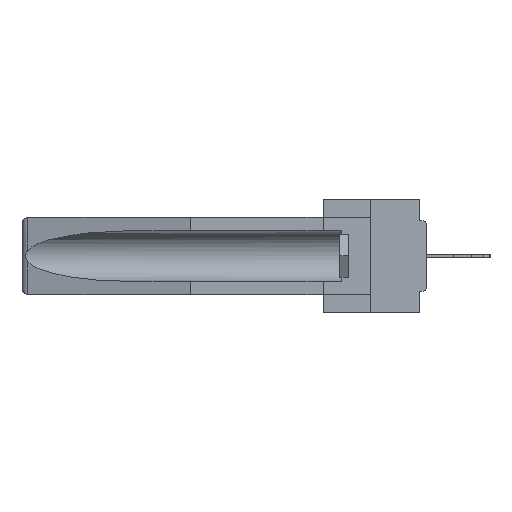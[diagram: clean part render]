
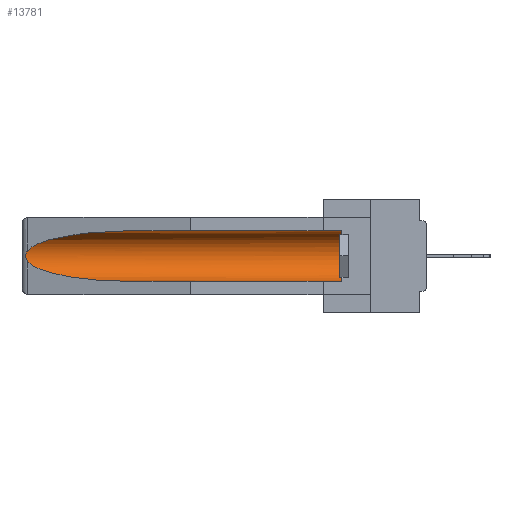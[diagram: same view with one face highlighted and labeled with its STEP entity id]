
A CAD part, left-side view. The second image highlights one B-rep face of the part: STEP entity #13781.
In plain terms, the highlighted cylindrical face has radius 2.857 mm (diameter 5.715 mm), a partial arc.
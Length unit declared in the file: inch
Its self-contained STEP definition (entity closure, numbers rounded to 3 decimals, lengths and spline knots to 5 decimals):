
#148 = CARTESIAN_POINT ( 'NONE',  ( 0.26597, 1.5296, -0.19026 ) ) ;
#657 = CARTESIAN_POINT ( 'NONE',  ( 0.155, 0.126, -0.284 ) ) ;
#1230 = DIRECTION ( 'NONE',  ( 0., 1., 0. ) ) ;
#2485 = AXIS2_PLACEMENT_3D ( 'NONE', #13371, #8374, #6191 ) ;
#3116 = VERTEX_POINT ( 'NONE', #3858 ) ;
#3160 = ORIENTED_EDGE ( 'NONE', *, *, #4886, .T. ) ;
#3295 = EDGE_CURVE ( 'NONE', #30971, #23489, #12190, .T. ) ;
#3858 = CARTESIAN_POINT ( 'NONE',  ( 0.26537, 1.52718, -0.19328 ) ) ;
#3945 = CARTESIAN_POINT ( 'NONE',  ( 0.21114, 1.30732, -0.059 ) ) ;
#4886 = EDGE_CURVE ( 'NONE', #3116, #23489, #19303, .T. ) ;
#5988 = CARTESIAN_POINT ( 'NONE',  ( 0.26654, 1.53092, -0.15636 ) ) ;
#6191 = DIRECTION ( 'NONE',  ( 0., 0., 1. ) ) ;
#6612 = CARTESIAN_POINT ( 'NONE',  ( 0.26537, 1.52718, -0.14972 ) ) ;
#7789 = CARTESIAN_POINT ( 'NONE',  ( 0.155, 1.07973, -0.059 ) ) ;
#8005 = CARTESIAN_POINT ( 'NONE',  ( 0.2675, 1.53308, -0.16763 ) ) ;
#8374 = DIRECTION ( 'NONE',  ( 0., -1., 0. ) ) ;
#8507 = CARTESIAN_POINT ( 'NONE',  ( 0.26655, 1.53094, -0.18657 ) ) ;
#8596 = CYLINDRICAL_SURFACE ( 'NONE', #26036, 0.1125 ) ;
#8895 = CIRCLE ( 'NONE', #2485, 0.1125 ) ;
#9211 = CARTESIAN_POINT ( 'NONE',  ( 0.155, 1.07973, -0.284 ) ) ;
#9322 = CARTESIAN_POINT ( 'NONE',  ( 0.155, 1.07973, -0.284 ) ) ;
#9360 = DIRECTION ( 'NONE',  ( 0., 1., 0. ) ) ;
#10658 = CARTESIAN_POINT ( 'NONE',  ( 0.26597, 1.52961, -0.15275 ) ) ;
#12055 = CARTESIAN_POINT ( 'NONE',  ( 0.155, -0.30754, -0.1715 ) ) ;
#12190 = LINE ( 'NONE', #16854, #20922 ) ;
#13371 = CARTESIAN_POINT ( 'NONE',  ( 0.155, 0.126, -0.1715 ) ) ;
#13781 = ADVANCED_FACE ( 'NONE', ( #31442 ), #8596, .F. ) ;
#13933 = CARTESIAN_POINT ( 'NONE',  ( 0.25451, 1.48313, -0.09465 ) ) ;
#13934 =( BOUNDED_CURVE ( )  B_SPLINE_CURVE ( 3, ( #16606, #3945, #13933, #6612 ),
 .UNSPECIFIED., .F., .T. ) 
 B_SPLINE_CURVE_WITH_KNOTS ( ( 4, 4 ),
 ( 4.71239, 6.08839 ),
 .UNSPECIFIED. ) 
 CURVE ( )  GEOMETRIC_REPRESENTATION_ITEM ( )  RATIONAL_B_SPLINE_CURVE ( ( 1., 0.848, 0.848, 1. ) ) 
 REPRESENTATION_ITEM ( '' )  );
#15101 = ORIENTED_EDGE ( 'NONE', *, *, #30493, .T. ) ;
#15494 = CARTESIAN_POINT ( 'NONE',  ( 0.2675, 1.53308, -0.17534 ) ) ;
#15659 = EDGE_LOOP ( 'NONE', ( #16030, #22967, #3160, #24551, #15101, #31260 ) ) ;
#16030 = ORIENTED_EDGE ( 'NONE', *, *, #25474, .T. ) ;
#16606 = CARTESIAN_POINT ( 'NONE',  ( 0.155, 1.07973, -0.059 ) ) ;
#16854 = CARTESIAN_POINT ( 'NONE',  ( 0.155, -0.30754, -0.284 ) ) ;
#17047 = CARTESIAN_POINT ( 'NONE',  ( 0.26537, 1.52718, -0.19328 ) ) ;
#18678 = CARTESIAN_POINT ( 'NONE',  ( 0.26537, 1.52718, -0.19328 ) ) ;
#19303 =( BOUNDED_CURVE ( )  B_SPLINE_CURVE ( 3, ( #17047, #24699, #26891, #9211 ),
 .UNSPECIFIED., .F., .T. ) 
 B_SPLINE_CURVE_WITH_KNOTS ( ( 4, 4 ),
 ( 0.1948, 1.5708 ),
 .UNSPECIFIED. ) 
 CURVE ( )  GEOMETRIC_REPRESENTATION_ITEM ( )  RATIONAL_B_SPLINE_CURVE ( ( 1., 0.848, 0.848, 1. ) ) 
 REPRESENTATION_ITEM ( '' )  );
#19989 = DIRECTION ( 'NONE',  ( 0., 1., 0. ) ) ;
#20922 = VECTOR ( 'NONE', #9360, 39.37008 ) ;
#22654 = LINE ( 'NONE', #27843, #30213 ) ;
#22967 = ORIENTED_EDGE ( 'NONE', *, *, #29733, .T. ) ;
#23489 = VERTEX_POINT ( 'NONE', #9322 ) ;
#23648 = EDGE_CURVE ( 'NONE', #31117, #28165, #22654, .T. ) ;
#24551 = ORIENTED_EDGE ( 'NONE', *, *, #3295, .F. ) ;
#24699 = CARTESIAN_POINT ( 'NONE',  ( 0.25451, 1.48313, -0.24835 ) ) ;
#25474 = EDGE_CURVE ( 'NONE', #28165, #28224, #13934, .T. ) ;
#26036 = AXIS2_PLACEMENT_3D ( 'NONE', #12055, #1230, #27255 ) ;
#26891 = CARTESIAN_POINT ( 'NONE',  ( 0.21114, 1.30732, -0.284 ) ) ;
#27255 = DIRECTION ( 'NONE',  ( 0., 0., 1. ) ) ;
#27843 = CARTESIAN_POINT ( 'NONE',  ( 0.155, -0.30754, -0.059 ) ) ;
#28165 = VERTEX_POINT ( 'NONE', #7789 ) ;
#28224 = VERTEX_POINT ( 'NONE', #30316 ) ;
#29733 = EDGE_CURVE ( 'NONE', #28224, #3116, #30189, .T. ) ;
#30189 = B_SPLINE_CURVE_WITH_KNOTS ( 'NONE', 3,
 ( #30848, #10658, #5988, #30994, #8005, #15494, #31343, #8507, #148, #18678 ),
 .UNSPECIFIED., .F., .F.,
 ( 4, 2, 2, 2, 4 ),
 ( 0., 0.00029, 0.00058, 0.00087, 0.00117 ),
 .UNSPECIFIED. ) ;
#30213 = VECTOR ( 'NONE', #19989, 39.37008 ) ;
#30316 = CARTESIAN_POINT ( 'NONE',  ( 0.26537, 1.52718, -0.14972 ) ) ;
#30493 = EDGE_CURVE ( 'NONE', #30971, #31117, #8895, .T. ) ;
#30848 = CARTESIAN_POINT ( 'NONE',  ( 0.26537, 1.52718, -0.14972 ) ) ;
#30971 = VERTEX_POINT ( 'NONE', #657 ) ;
#30994 = CARTESIAN_POINT ( 'NONE',  ( 0.2673, 1.5327, -0.16383 ) ) ;
#31117 = VERTEX_POINT ( 'NONE', #31828 ) ;
#31260 = ORIENTED_EDGE ( 'NONE', *, *, #23648, .T. ) ;
#31343 = CARTESIAN_POINT ( 'NONE',  ( 0.2673, 1.53269, -0.17917 ) ) ;
#31442 = FACE_OUTER_BOUND ( 'NONE', #15659, .T. ) ;
#31828 = CARTESIAN_POINT ( 'NONE',  ( 0.155, 0.126, -0.059 ) ) ;
